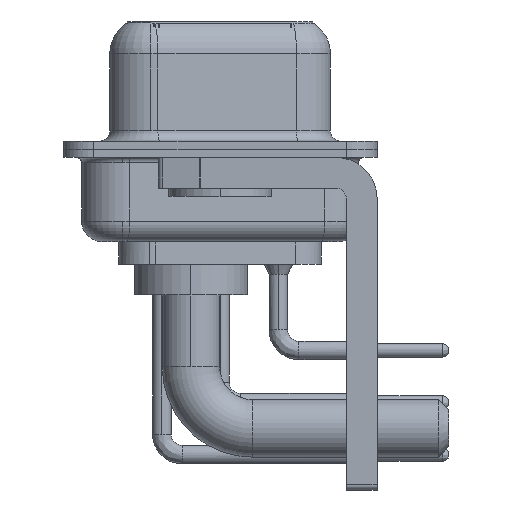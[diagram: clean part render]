
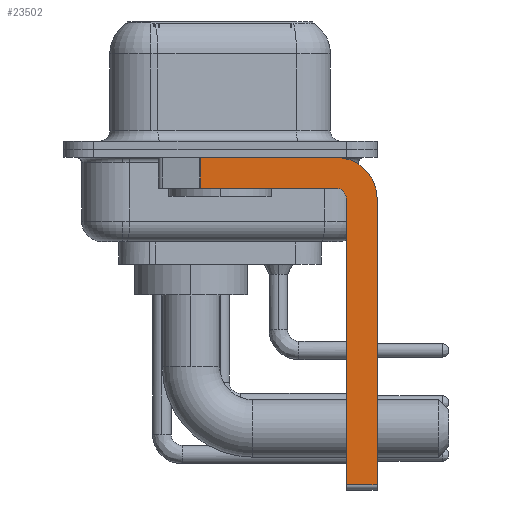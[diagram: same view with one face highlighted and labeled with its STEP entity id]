
A CAD part, left-side view. The second image highlights one B-rep face of the part: STEP entity #23502.
In plain terms, the highlighted planar face has unit normal (-1, 0, 0).
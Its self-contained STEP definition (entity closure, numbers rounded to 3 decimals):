
#273 = EDGE_CURVE ( 'NONE', #4696, #20591, #26347, .T. ) ;
#590 = CARTESIAN_POINT ( 'NONE',  ( -2.9, -5.65, -2.4 ) ) ;
#852 = EDGE_CURVE ( 'NONE', #26757, #20664, #29991, .T. ) ;
#924 = AXIS2_PLACEMENT_3D ( 'NONE', #590, #11116, #8820 ) ;
#1870 = DIRECTION ( 'NONE',  ( 1., 0., 0. ) ) ;
#2089 = EDGE_LOOP ( 'NONE', ( #3379, #32189, #2328, #27602, #17448, #8645, #18640, #29347 ) ) ;
#2316 = DIRECTION ( 'NONE',  ( 0., 1., 0. ) ) ;
#2328 = ORIENTED_EDGE ( 'NONE', *, *, #273, .F. ) ;
#3280 = CARTESIAN_POINT ( 'NONE',  ( -2.9, -7.65, -2.4 ) ) ;
#3379 = ORIENTED_EDGE ( 'NONE', *, *, #25255, .F. ) ;
#4696 = VERTEX_POINT ( 'NONE', #13926 ) ;
#4888 = CARTESIAN_POINT ( 'NONE',  ( -2.9, -5.65, -16.35 ) ) ;
#5794 = VECTOR ( 'NONE', #5889, 1000. ) ;
#5889 = DIRECTION ( 'NONE',  ( 0., 0., -1. ) ) ;
#6418 = VERTEX_POINT ( 'NONE', #23461 ) ;
#7162 = CARTESIAN_POINT ( 'NONE',  ( -2.9, -7.65, -2.4 ) ) ;
#7402 = AXIS2_PLACEMENT_3D ( 'NONE', #16327, #24575, #22289 ) ;
#8645 = ORIENTED_EDGE ( 'NONE', *, *, #14939, .T. ) ;
#8820 = DIRECTION ( 'NONE',  ( 0., 0., -1. ) ) ;
#9137 = LINE ( 'NONE', #11777, #22782 ) ;
#10041 = EDGE_CURVE ( 'NONE', #26582, #20591, #18655, .T. ) ;
#10148 = DIRECTION ( 'NONE',  ( 0., -1., 0. ) ) ;
#10469 = VECTOR ( 'NONE', #10148, 1000. ) ;
#11116 = DIRECTION ( 'NONE',  ( 1., 0., 0. ) ) ;
#11730 = LINE ( 'NONE', #11896, #14474 ) ;
#11777 = CARTESIAN_POINT ( 'NONE',  ( -2.9, -6.15, -16.6 ) ) ;
#11896 = CARTESIAN_POINT ( 'NONE',  ( -2.9, 3., -0.4 ) ) ;
#12507 = VECTOR ( 'NONE', #2316, 1000. ) ;
#13926 = CARTESIAN_POINT ( 'NONE',  ( -2.9, -5.65, -1.9 ) ) ;
#14474 = VECTOR ( 'NONE', #32483, 1000. ) ;
#14544 = CARTESIAN_POINT ( 'NONE',  ( -2.9, 0.978, -0.4 ) ) ;
#14939 = EDGE_CURVE ( 'NONE', #21616, #20664, #21023, .T. ) ;
#14998 = EDGE_CURVE ( 'NONE', #21616, #21188, #9137, .T. ) ;
#15709 = DIRECTION ( 'NONE',  ( 0., 0., -1. ) ) ;
#16327 = CARTESIAN_POINT ( 'NONE',  ( -2.9, -5.65, -2.4 ) ) ;
#17105 = CARTESIAN_POINT ( 'NONE',  ( -2.9, -6.15, -16.35 ) ) ;
#17410 = DIRECTION ( 'NONE',  ( 0., 0., 1. ) ) ;
#17448 = ORIENTED_EDGE ( 'NONE', *, *, #14998, .F. ) ;
#18640 = ORIENTED_EDGE ( 'NONE', *, *, #852, .F. ) ;
#18655 = LINE ( 'NONE', #32536, #24609 ) ;
#19781 = CIRCLE ( 'NONE', #28188, 2. ) ;
#20591 = VERTEX_POINT ( 'NONE', #29592 ) ;
#20664 = VERTEX_POINT ( 'NONE', #24640 ) ;
#21023 = LINE ( 'NONE', #4888, #10469 ) ;
#21188 = VERTEX_POINT ( 'NONE', #32530 ) ;
#21616 = VERTEX_POINT ( 'NONE', #17105 ) ;
#22289 = DIRECTION ( 'NONE',  ( 0., 0., 1. ) ) ;
#22676 = EDGE_CURVE ( 'NONE', #21188, #4696, #24212, .T. ) ;
#22782 = VECTOR ( 'NONE', #17410, 1000. ) ;
#23461 = CARTESIAN_POINT ( 'NONE',  ( -2.9, -5.65, -0.4 ) ) ;
#23502 = ADVANCED_FACE ( 'NONE', ( #34351 ), #24980, .F. ) ;
#23784 = CARTESIAN_POINT ( 'NONE',  ( -2.9, -5.65, -2.4 ) ) ;
#24212 = CIRCLE ( 'NONE', #7402, 0.5 ) ;
#24575 = DIRECTION ( 'NONE',  ( -1., 0., 0. ) ) ;
#24609 = VECTOR ( 'NONE', #32187, 1000. ) ;
#24640 = CARTESIAN_POINT ( 'NONE',  ( -2.9, -7.65, -16.35 ) ) ;
#24980 = PLANE ( 'NONE',  #924 ) ;
#25255 = EDGE_CURVE ( 'NONE', #26582, #6418, #11730, .T. ) ;
#26347 = LINE ( 'NONE', #26515, #12507 ) ;
#26515 = CARTESIAN_POINT ( 'NONE',  ( -2.9, -5.65, -1.9 ) ) ;
#26582 = VERTEX_POINT ( 'NONE', #14544 ) ;
#26757 = VERTEX_POINT ( 'NONE', #7162 ) ;
#27602 = ORIENTED_EDGE ( 'NONE', *, *, #22676, .F. ) ;
#28188 = AXIS2_PLACEMENT_3D ( 'NONE', #23784, #1870, #15709 ) ;
#29347 = ORIENTED_EDGE ( 'NONE', *, *, #33786, .F. ) ;
#29592 = CARTESIAN_POINT ( 'NONE',  ( -2.9, 0.978, -1.9 ) ) ;
#29991 = LINE ( 'NONE', #3280, #5794 ) ;
#32187 = DIRECTION ( 'NONE',  ( 0., 0., -1. ) ) ;
#32189 = ORIENTED_EDGE ( 'NONE', *, *, #10041, .T. ) ;
#32483 = DIRECTION ( 'NONE',  ( 0., -1., 0. ) ) ;
#32530 = CARTESIAN_POINT ( 'NONE',  ( -2.9, -6.15, -2.4 ) ) ;
#32536 = CARTESIAN_POINT ( 'NONE',  ( -2.9, 0.978, -1.9 ) ) ;
#33786 = EDGE_CURVE ( 'NONE', #6418, #26757, #19781, .T. ) ;
#34351 = FACE_OUTER_BOUND ( 'NONE', #2089, .T. ) ;
